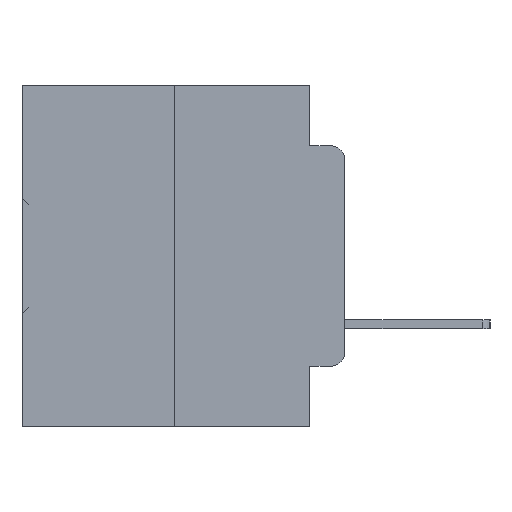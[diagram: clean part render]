
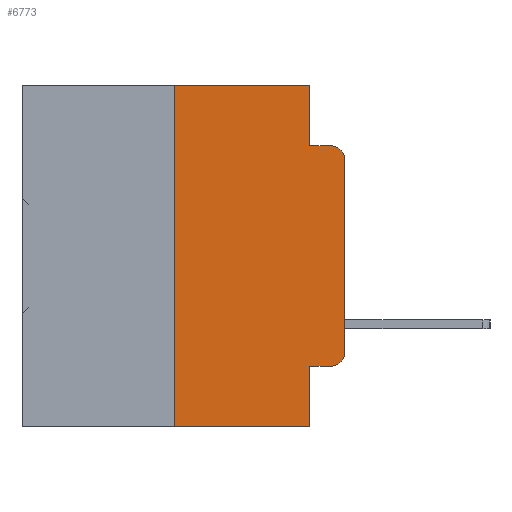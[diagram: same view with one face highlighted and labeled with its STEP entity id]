
A CAD part, left-side view. The second image highlights one B-rep face of the part: STEP entity #6773.
In plain terms, the highlighted planar face has unit normal (-1, 0, 0).
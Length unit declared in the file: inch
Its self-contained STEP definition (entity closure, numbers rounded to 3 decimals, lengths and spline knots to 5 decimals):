
#762 = EDGE_CURVE ( 'NONE', #1179, #26140, #11868, .T. ) ;
#808 = EDGE_CURVE ( 'NONE', #13314, #1179, #26230, .T. ) ;
#1179 = VERTEX_POINT ( 'NONE', #19218 ) ;
#1732 = CIRCLE ( 'NONE', #31679, 0.02 ) ;
#2587 = CARTESIAN_POINT ( 'NONE',  ( 0., 0.051, -0.0885 ) ) ;
#2588 = EDGE_CURVE ( 'NONE', #26140, #3316, #11727, .T. ) ;
#2979 = ORIENTED_EDGE ( 'NONE', *, *, #2588, .F. ) ;
#3316 = VERTEX_POINT ( 'NONE', #5179 ) ;
#3744 = CARTESIAN_POINT ( 'NONE',  ( 0., 0.25, 0. ) ) ;
#3815 = ORIENTED_EDGE ( 'NONE', *, *, #23422, .T. ) ;
#4192 = CARTESIAN_POINT ( 'NONE',  ( 0., 0.473, -0.5 ) ) ;
#4330 = ORIENTED_EDGE ( 'NONE', *, *, #32738, .T. ) ;
#4343 = AXIS2_PLACEMENT_3D ( 'NONE', #9972, #28851, #12762 ) ;
#4433 = DIRECTION ( 'NONE',  ( 0., 0., -1. ) ) ;
#4442 = EDGE_CURVE ( 'NONE', #34495, #3316, #29637, .T. ) ;
#4681 = ORIENTED_EDGE ( 'NONE', *, *, #25217, .T. ) ;
#5179 = CARTESIAN_POINT ( 'NONE',  ( 0., 0.02, -0.0885 ) ) ;
#6001 = ORIENTED_EDGE ( 'NONE', *, *, #32276, .F. ) ;
#6171 = CARTESIAN_POINT ( 'NONE',  ( 0., 0.051, -0.4115 ) ) ;
#6194 = LINE ( 'NONE', #11845, #26653 ) ;
#6773 = ADVANCED_FACE ( 'NONE', ( #11728 ), #26199, .F. ) ;
#7221 = CARTESIAN_POINT ( 'NONE',  ( 0., 0.25, -0.5 ) ) ;
#7709 = CARTESIAN_POINT ( 'NONE',  ( 0., 0.051, -0.4115 ) ) ;
#7746 = DIRECTION ( 'NONE',  ( 0., 0., -1. ) ) ;
#8178 = CARTESIAN_POINT ( 'NONE',  ( 0., 0.051, -0.5 ) ) ;
#8179 = EDGE_CURVE ( 'NONE', #29301, #34495, #16759, .T. ) ;
#8397 = VERTEX_POINT ( 'NONE', #7709 ) ;
#9017 = CARTESIAN_POINT ( 'NONE',  ( 0., 0., -0.3915 ) ) ;
#9199 = EDGE_LOOP ( 'NONE', ( #30505, #27668, #2979, #26830, #18822, #6001, #4330, #12894, #4681, #3815 ) ) ;
#9972 = CARTESIAN_POINT ( 'NONE',  ( 0., 0.473, 0. ) ) ;
#10841 = VECTOR ( 'NONE', #14293, 39.37008 ) ;
#10984 = VECTOR ( 'NONE', #27174, 39.37008 ) ;
#11727 = LINE ( 'NONE', #24392, #10841 ) ;
#11728 = FACE_OUTER_BOUND ( 'NONE', #9199, .T. ) ;
#11845 = CARTESIAN_POINT ( 'NONE',  ( 0., 0.051, 0. ) ) ;
#11868 = LINE ( 'NONE', #17497, #12734 ) ;
#12734 = VECTOR ( 'NONE', #4433, 39.37008 ) ;
#12762 = DIRECTION ( 'NONE',  ( 0., 0., -1. ) ) ;
#12894 = ORIENTED_EDGE ( 'NONE', *, *, #27005, .F. ) ;
#13314 = VERTEX_POINT ( 'NONE', #3744 ) ;
#13842 = VECTOR ( 'NONE', #34622, 39.37008 ) ;
#14293 = DIRECTION ( 'NONE',  ( 0., -1., 0. ) ) ;
#14709 = DIRECTION ( 'NONE',  ( -1., 0., 0. ) ) ;
#16759 = LINE ( 'NONE', #18677, #30141 ) ;
#17497 = CARTESIAN_POINT ( 'NONE',  ( 0., 0.051, 0. ) ) ;
#18677 = CARTESIAN_POINT ( 'NONE',  ( 0., 0., 0. ) ) ;
#18822 = ORIENTED_EDGE ( 'NONE', *, *, #808, .F. ) ;
#19218 = CARTESIAN_POINT ( 'NONE',  ( 0., 0.051, 0. ) ) ;
#19712 = DIRECTION ( 'NONE',  ( -1., 0., 0. ) ) ;
#20846 = VECTOR ( 'NONE', #30494, 39.37008 ) ;
#21867 = LINE ( 'NONE', #26706, #13842 ) ;
#21918 = CARTESIAN_POINT ( 'NONE',  ( 0., 0., -0.1085 ) ) ;
#23422 = EDGE_CURVE ( 'NONE', #27545, #29301, #1732, .T. ) ;
#24392 = CARTESIAN_POINT ( 'NONE',  ( 0., 0.051, -0.0885 ) ) ;
#25217 = EDGE_CURVE ( 'NONE', #8397, #27545, #27972, .T. ) ;
#25954 = VERTEX_POINT ( 'NONE', #7221 ) ;
#25986 = DIRECTION ( 'NONE',  ( 0., -1., 0. ) ) ;
#26140 = VERTEX_POINT ( 'NONE', #2587 ) ;
#26161 = VERTEX_POINT ( 'NONE', #8178 ) ;
#26199 = PLANE ( 'NONE',  #4343 ) ;
#26230 = LINE ( 'NONE', #29197, #10984 ) ;
#26460 = VECTOR ( 'NONE', #25986, 39.37008 ) ;
#26653 = VECTOR ( 'NONE', #27991, 39.37008 ) ;
#26706 = CARTESIAN_POINT ( 'NONE',  ( 0., 0.25, 0. ) ) ;
#26830 = ORIENTED_EDGE ( 'NONE', *, *, #762, .F. ) ;
#27005 = EDGE_CURVE ( 'NONE', #8397, #26161, #6194, .T. ) ;
#27174 = DIRECTION ( 'NONE',  ( 0., -1., 0. ) ) ;
#27295 = LINE ( 'NONE', #4192, #26460 ) ;
#27545 = VERTEX_POINT ( 'NONE', #30462 ) ;
#27668 = ORIENTED_EDGE ( 'NONE', *, *, #4442, .T. ) ;
#27972 = LINE ( 'NONE', #6171, #20846 ) ;
#27991 = DIRECTION ( 'NONE',  ( 0., 0., -1. ) ) ;
#28506 = CARTESIAN_POINT ( 'NONE',  ( 0., 0.02, -0.1085 ) ) ;
#28851 = DIRECTION ( 'NONE',  ( 1., 0., 0. ) ) ;
#29197 = CARTESIAN_POINT ( 'NONE',  ( 0., 0.473, 0. ) ) ;
#29301 = VERTEX_POINT ( 'NONE', #9017 ) ;
#29637 = CIRCLE ( 'NONE', #29690, 0.02 ) ;
#29690 = AXIS2_PLACEMENT_3D ( 'NONE', #28506, #19712, #7746 ) ;
#30141 = VECTOR ( 'NONE', #34604, 39.37008 ) ;
#30462 = CARTESIAN_POINT ( 'NONE',  ( 0., 0.02, -0.4115 ) ) ;
#30494 = DIRECTION ( 'NONE',  ( 0., -1., 0. ) ) ;
#30505 = ORIENTED_EDGE ( 'NONE', *, *, #8179, .T. ) ;
#30720 = CARTESIAN_POINT ( 'NONE',  ( 0., 0.02, -0.3915 ) ) ;
#31679 = AXIS2_PLACEMENT_3D ( 'NONE', #30720, #14709, #33377 ) ;
#32276 = EDGE_CURVE ( 'NONE', #25954, #13314, #21867, .T. ) ;
#32738 = EDGE_CURVE ( 'NONE', #25954, #26161, #27295, .T. ) ;
#33377 = DIRECTION ( 'NONE',  ( 0., 0., -1. ) ) ;
#34495 = VERTEX_POINT ( 'NONE', #21918 ) ;
#34604 = DIRECTION ( 'NONE',  ( 0., 0., 1. ) ) ;
#34622 = DIRECTION ( 'NONE',  ( 0., 0., 1. ) ) ;
